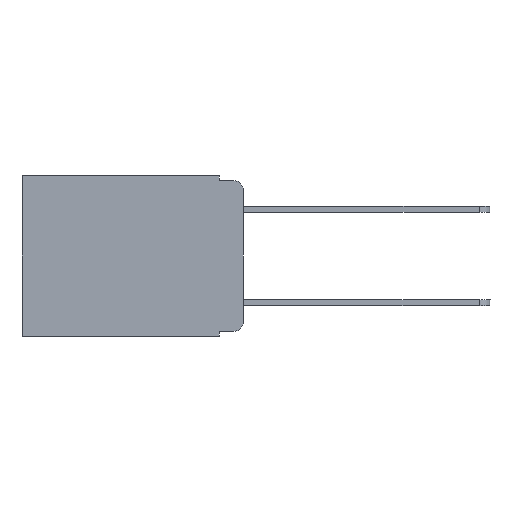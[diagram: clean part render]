
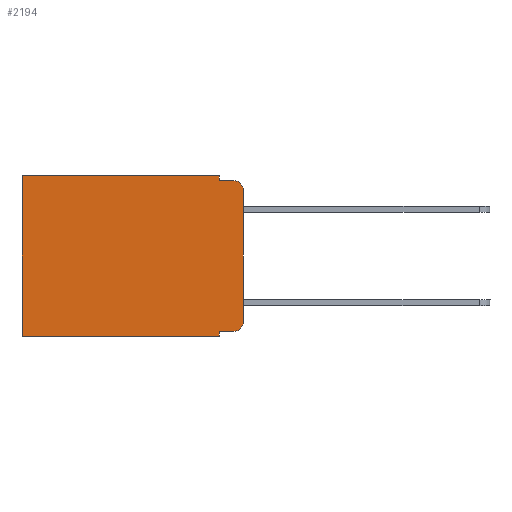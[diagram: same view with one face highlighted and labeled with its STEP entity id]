
A CAD part, left-side view. The second image highlights one B-rep face of the part: STEP entity #2194.
In plain terms, the highlighted planar face has unit normal (-1, 0, 0).
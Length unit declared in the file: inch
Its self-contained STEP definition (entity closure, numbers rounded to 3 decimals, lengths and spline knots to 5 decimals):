
#38 = CARTESIAN_POINT ( 'NONE',  ( 0.298, 0.051, 0. ) ) ;
#191 = CARTESIAN_POINT ( 'NONE',  ( 0.298, 0., 0. ) ) ;
#212 = DIRECTION ( 'NONE',  ( -1., 0., 0. ) ) ;
#905 = FACE_OUTER_BOUND ( 'NONE', #929, .T. ) ;
#907 = CARTESIAN_POINT ( 'NONE',  ( 0.298, 0., -0.313 ) ) ;
#929 = EDGE_LOOP ( 'NONE', ( #6114, #1939, #1916, #5762, #7670, #6224, #3630, #5681, #5219, #4838 ) ) ;
#1011 = DIRECTION ( 'NONE',  ( 0., 1., 0. ) ) ;
#1393 = VECTOR ( 'NONE', #7376, 39.37008 ) ;
#1437 = CARTESIAN_POINT ( 'NONE',  ( 0.298, 0., -0.03 ) ) ;
#1518 = CARTESIAN_POINT ( 'NONE',  ( 0.298, 0.051, -0.01 ) ) ;
#1772 = CARTESIAN_POINT ( 'NONE',  ( 0.298, 0., 0. ) ) ;
#1798 = CARTESIAN_POINT ( 'NONE',  ( 0.298, 0.051, -0.343 ) ) ;
#1916 = ORIENTED_EDGE ( 'NONE', *, *, #9245, .F. ) ;
#1939 = ORIENTED_EDGE ( 'NONE', *, *, #8015, .T. ) ;
#2055 = VECTOR ( 'NONE', #6812, 39.37008 ) ;
#2101 = VERTEX_POINT ( 'NONE', #6671 ) ;
#2135 = CARTESIAN_POINT ( 'NONE',  ( 0.298, 0.051, -0.01 ) ) ;
#2187 = CARTESIAN_POINT ( 'NONE',  ( 0.298, 0.02, -0.313 ) ) ;
#2194 = ADVANCED_FACE ( 'NONE', ( #905 ), #6757, .F. ) ;
#2247 = DIRECTION ( 'NONE',  ( 0., 0., -1. ) ) ;
#2281 = CARTESIAN_POINT ( 'NONE',  ( 0.298, 0.473, 0. ) ) ;
#2332 = AXIS2_PLACEMENT_3D ( 'NONE', #6784, #212, #4475 ) ;
#2491 = VERTEX_POINT ( 'NONE', #1437 ) ;
#2861 = DIRECTION ( 'NONE',  ( -1., 0., 0. ) ) ;
#3105 = DIRECTION ( 'NONE',  ( 1., 0., 0. ) ) ;
#3193 = VECTOR ( 'NONE', #8289, 39.37008 ) ;
#3253 = CARTESIAN_POINT ( 'NONE',  ( 0.298, 0., -0.343 ) ) ;
#3572 = DIRECTION ( 'NONE',  ( 0., -1., 0. ) ) ;
#3629 = LINE ( 'NONE', #38, #1393 ) ;
#3630 = ORIENTED_EDGE ( 'NONE', *, *, #6719, .F. ) ;
#3918 = DIRECTION ( 'NONE',  ( 0., 0., -1. ) ) ;
#4475 = DIRECTION ( 'NONE',  ( 0., 0., -1. ) ) ;
#4598 = LINE ( 'NONE', #3253, #5029 ) ;
#4646 = VERTEX_POINT ( 'NONE', #8113 ) ;
#4827 = VECTOR ( 'NONE', #3918, 39.37008 ) ;
#4838 = ORIENTED_EDGE ( 'NONE', *, *, #8784, .T. ) ;
#5024 = DIRECTION ( 'NONE',  ( 0., 0., -1. ) ) ;
#5029 = VECTOR ( 'NONE', #1011, 39.37008 ) ;
#5030 = VERTEX_POINT ( 'NONE', #7778 ) ;
#5210 = VERTEX_POINT ( 'NONE', #907 ) ;
#5219 = ORIENTED_EDGE ( 'NONE', *, *, #6659, .T. ) ;
#5231 = EDGE_CURVE ( 'NONE', #4646, #7451, #8930, .T. ) ;
#5258 = VERTEX_POINT ( 'NONE', #8242 ) ;
#5350 = CARTESIAN_POINT ( 'NONE',  ( 0.298, 0.051, 0. ) ) ;
#5381 = AXIS2_PLACEMENT_3D ( 'NONE', #191, #3105, #2247 ) ;
#5428 = CIRCLE ( 'NONE', #8822, 0.02 ) ;
#5637 = VECTOR ( 'NONE', #8249, 39.37008 ) ;
#5681 = ORIENTED_EDGE ( 'NONE', *, *, #7123, .F. ) ;
#5762 = ORIENTED_EDGE ( 'NONE', *, *, #7481, .F. ) ;
#5775 = LINE ( 'NONE', #1518, #9179 ) ;
#5797 = EDGE_CURVE ( 'NONE', #7451, #5258, #5988, .T. ) ;
#5988 = LINE ( 'NONE', #6755, #4827 ) ;
#6114 = ORIENTED_EDGE ( 'NONE', *, *, #7000, .F. ) ;
#6160 = CARTESIAN_POINT ( 'NONE',  ( 0.298, 0.051, -0.333 ) ) ;
#6224 = ORIENTED_EDGE ( 'NONE', *, *, #5797, .T. ) ;
#6476 = CIRCLE ( 'NONE', #2332, 0.02 ) ;
#6659 = EDGE_CURVE ( 'NONE', #9355, #2101, #8386, .T. ) ;
#6671 = CARTESIAN_POINT ( 'NONE',  ( 0.298, 0.02, -0.333 ) ) ;
#6719 = EDGE_CURVE ( 'NONE', #7667, #5258, #4598, .T. ) ;
#6755 = CARTESIAN_POINT ( 'NONE',  ( 0.298, 0.473, 0. ) ) ;
#6757 = PLANE ( 'NONE',  #5381 ) ;
#6784 = CARTESIAN_POINT ( 'NONE',  ( 0.298, 0.02, -0.03 ) ) ;
#6812 = DIRECTION ( 'NONE',  ( 0., 1., 0. ) ) ;
#6856 = LINE ( 'NONE', #5350, #3193 ) ;
#7000 = EDGE_CURVE ( 'NONE', #2491, #5210, #8098, .T. ) ;
#7123 = EDGE_CURVE ( 'NONE', #9355, #7667, #6856, .T. ) ;
#7376 = DIRECTION ( 'NONE',  ( 0., 0., -1. ) ) ;
#7420 = DIRECTION ( 'NONE',  ( 0., 0., -1. ) ) ;
#7451 = VERTEX_POINT ( 'NONE', #2281 ) ;
#7481 = EDGE_CURVE ( 'NONE', #4646, #7503, #3629, .T. ) ;
#7503 = VERTEX_POINT ( 'NONE', #2135 ) ;
#7667 = VERTEX_POINT ( 'NONE', #1798 ) ;
#7670 = ORIENTED_EDGE ( 'NONE', *, *, #5231, .T. ) ;
#7778 = CARTESIAN_POINT ( 'NONE',  ( 0.298, 0.02, -0.01 ) ) ;
#7952 = CARTESIAN_POINT ( 'NONE',  ( 0.298, 0., 0. ) ) ;
#8015 = EDGE_CURVE ( 'NONE', #2491, #5030, #6476, .T. ) ;
#8098 = LINE ( 'NONE', #7952, #8565 ) ;
#8113 = CARTESIAN_POINT ( 'NONE',  ( 0.298, 0.051, 0. ) ) ;
#8242 = CARTESIAN_POINT ( 'NONE',  ( 0.298, 0.473, -0.343 ) ) ;
#8249 = DIRECTION ( 'NONE',  ( 0., -1., 0. ) ) ;
#8289 = DIRECTION ( 'NONE',  ( 0., 0., -1. ) ) ;
#8344 = CARTESIAN_POINT ( 'NONE',  ( 0.298, 0.051, -0.333 ) ) ;
#8386 = LINE ( 'NONE', #8344, #5637 ) ;
#8565 = VECTOR ( 'NONE', #5024, 39.37008 ) ;
#8784 = EDGE_CURVE ( 'NONE', #2101, #5210, #5428, .T. ) ;
#8822 = AXIS2_PLACEMENT_3D ( 'NONE', #2187, #2861, #7420 ) ;
#8930 = LINE ( 'NONE', #1772, #2055 ) ;
#9179 = VECTOR ( 'NONE', #3572, 39.37008 ) ;
#9245 = EDGE_CURVE ( 'NONE', #7503, #5030, #5775, .T. ) ;
#9355 = VERTEX_POINT ( 'NONE', #6160 ) ;
